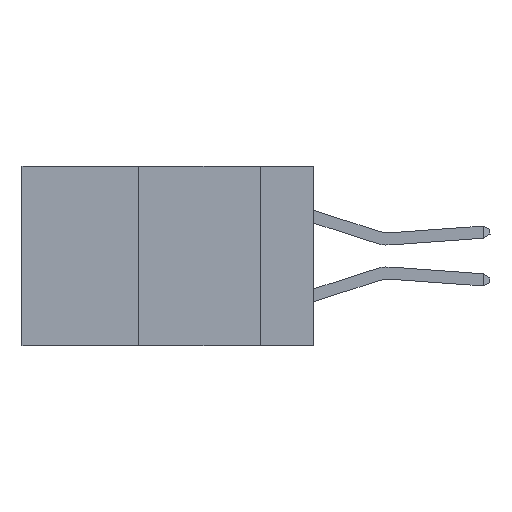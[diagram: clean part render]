
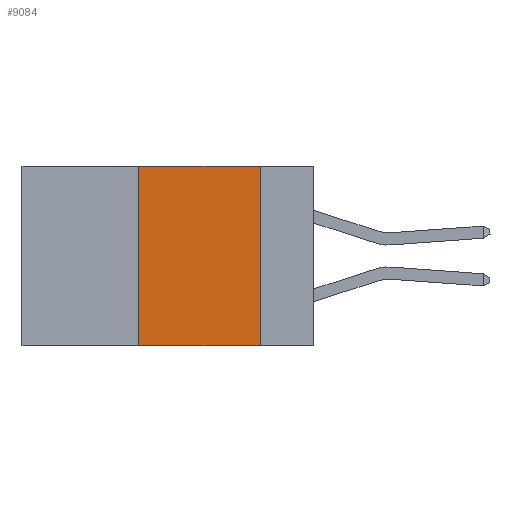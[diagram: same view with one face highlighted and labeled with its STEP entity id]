
A CAD part, left-side view. The second image highlights one B-rep face of the part: STEP entity #9084.
In plain terms, the highlighted planar face has unit normal (-1, 0, 0).
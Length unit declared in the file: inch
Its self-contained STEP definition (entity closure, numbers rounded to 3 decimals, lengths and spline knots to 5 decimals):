
#384 = LINE ( 'NONE', #1053, #21812 ) ;
#1053 = CARTESIAN_POINT ( 'NONE',  ( 0., 0.6, 0. ) ) ;
#1857 = ORIENTED_EDGE ( 'NONE', *, *, #18287, .F. ) ;
#3127 = EDGE_CURVE ( 'NONE', #20755, #14224, #16080, .T. ) ;
#3989 = EDGE_CURVE ( 'NONE', #18323, #14224, #32638, .T. ) ;
#4277 = PLANE ( 'NONE',  #20464 ) ;
#4442 = LINE ( 'NONE', #22141, #23803 ) ;
#4731 = DIRECTION ( 'NONE',  ( 0., 0., -1. ) ) ;
#7021 = ORIENTED_EDGE ( 'NONE', *, *, #3127, .F. ) ;
#9084 = ADVANCED_FACE ( 'NONE', ( #29631 ), #4277, .F. ) ;
#9597 = CARTESIAN_POINT ( 'NONE',  ( 0., 0.11, -0.37 ) ) ;
#9804 = CARTESIAN_POINT ( 'NONE',  ( 0., 0.6, -0.37 ) ) ;
#10590 = ORIENTED_EDGE ( 'NONE', *, *, #3989, .T. ) ;
#13117 = DIRECTION ( 'NONE',  ( 0., -1., 0. ) ) ;
#14224 = VERTEX_POINT ( 'NONE', #9597 ) ;
#15740 = CARTESIAN_POINT ( 'NONE',  ( 0., 0.11, 0. ) ) ;
#15902 = VERTEX_POINT ( 'NONE', #17392 ) ;
#16080 = LINE ( 'NONE', #15740, #30586 ) ;
#17287 = CARTESIAN_POINT ( 'NONE',  ( 0., 0.6, 0. ) ) ;
#17392 = CARTESIAN_POINT ( 'NONE',  ( 0., 0.36, 0. ) ) ;
#17463 = DIRECTION ( 'NONE',  ( 0., -1., 0. ) ) ;
#18287 = EDGE_CURVE ( 'NONE', #18323, #15902, #4442, .T. ) ;
#18323 = VERTEX_POINT ( 'NONE', #27939 ) ;
#19321 = VECTOR ( 'NONE', #17463, 39.37008 ) ;
#20105 = DIRECTION ( 'NONE',  ( 1., 0., 0. ) ) ;
#20444 = ORIENTED_EDGE ( 'NONE', *, *, #24115, .F. ) ;
#20464 = AXIS2_PLACEMENT_3D ( 'NONE', #17287, #20105, #4731 ) ;
#20755 = VERTEX_POINT ( 'NONE', #28699 ) ;
#21812 = VECTOR ( 'NONE', #13117, 39.37008 ) ;
#22141 = CARTESIAN_POINT ( 'NONE',  ( 0., 0.36, 0. ) ) ;
#23072 = DIRECTION ( 'NONE',  ( 0., 0., -1. ) ) ;
#23803 = VECTOR ( 'NONE', #32307, 39.37008 ) ;
#24115 = EDGE_CURVE ( 'NONE', #15902, #20755, #384, .T. ) ;
#26239 = EDGE_LOOP ( 'NONE', ( #7021, #20444, #1857, #10590 ) ) ;
#27939 = CARTESIAN_POINT ( 'NONE',  ( 0., 0.36, -0.37 ) ) ;
#28699 = CARTESIAN_POINT ( 'NONE',  ( 0., 0.11, 0. ) ) ;
#29631 = FACE_OUTER_BOUND ( 'NONE', #26239, .T. ) ;
#30586 = VECTOR ( 'NONE', #23072, 39.37008 ) ;
#32307 = DIRECTION ( 'NONE',  ( 0., 0., 1. ) ) ;
#32638 = LINE ( 'NONE', #9804, #19321 ) ;
